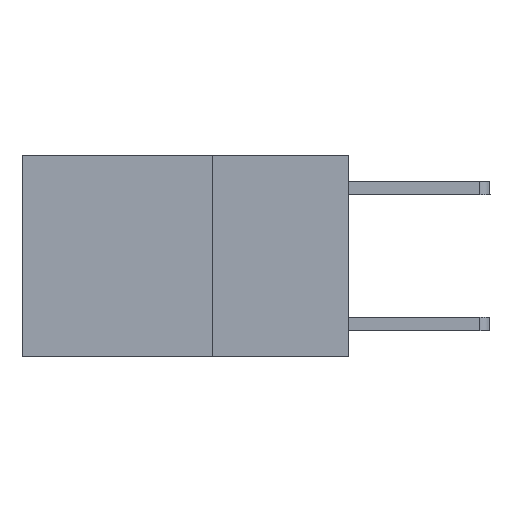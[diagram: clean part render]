
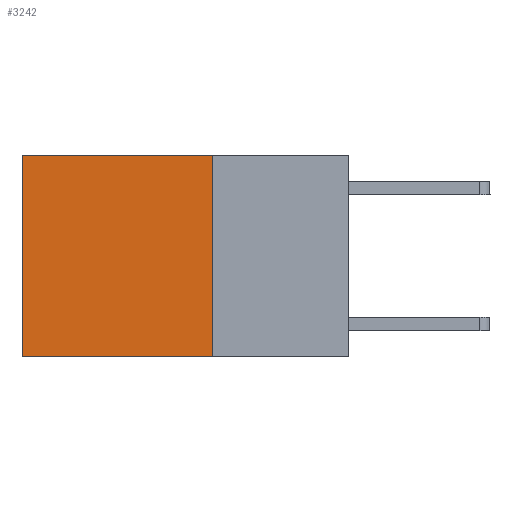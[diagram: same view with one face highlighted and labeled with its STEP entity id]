
A CAD part, left-side view. The second image highlights one B-rep face of the part: STEP entity #3242.
In plain terms, the highlighted planar face has unit normal (-1, 0, 0).
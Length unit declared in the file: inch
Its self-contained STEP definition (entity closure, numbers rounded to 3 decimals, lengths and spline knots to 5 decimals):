
#153 = VECTOR ( 'NONE', #1474, 39.37008 ) ;
#542 = CARTESIAN_POINT ( 'NONE',  ( 0.2625, 0.6, 0. ) ) ;
#686 = VERTEX_POINT ( 'NONE', #6622 ) ;
#793 = EDGE_CURVE ( 'NONE', #686, #1747, #1711, .T. ) ;
#1313 = AXIS2_PLACEMENT_3D ( 'NONE', #2365, #9253, #4961 ) ;
#1388 = LINE ( 'NONE', #542, #5122 ) ;
#1440 = EDGE_CURVE ( 'NONE', #686, #9752, #7326, .T. ) ;
#1474 = DIRECTION ( 'NONE',  ( 0., 1., 0. ) ) ;
#1711 = LINE ( 'NONE', #1775, #5719 ) ;
#1747 = VERTEX_POINT ( 'NONE', #4482 ) ;
#1775 = CARTESIAN_POINT ( 'NONE',  ( 0.2625, 0.25, 0. ) ) ;
#2359 = EDGE_CURVE ( 'NONE', #9752, #10469, #1388, .T. ) ;
#2365 = CARTESIAN_POINT ( 'NONE',  ( 0.2625, 0.25, 0. ) ) ;
#2575 = ORIENTED_EDGE ( 'NONE', *, *, #9671, .F. ) ;
#2678 = ORIENTED_EDGE ( 'NONE', *, *, #793, .F. ) ;
#2779 = DIRECTION ( 'NONE',  ( 0., 0., -1. ) ) ;
#3090 = DIRECTION ( 'NONE',  ( 0., 1., 0. ) ) ;
#3240 = LINE ( 'NONE', #7559, #153 ) ;
#3242 = ADVANCED_FACE ( 'NONE', ( #11192 ), #10095, .F. ) ;
#4482 = CARTESIAN_POINT ( 'NONE',  ( 0.2625, 0.25, -0.37 ) ) ;
#4822 = CARTESIAN_POINT ( 'NONE',  ( 0.2625, 0.25, 0. ) ) ;
#4961 = DIRECTION ( 'NONE',  ( 0., 0., -1. ) ) ;
#5122 = VECTOR ( 'NONE', #2779, 39.37008 ) ;
#5719 = VECTOR ( 'NONE', #6914, 39.37008 ) ;
#6073 = ORIENTED_EDGE ( 'NONE', *, *, #2359, .T. ) ;
#6189 = CARTESIAN_POINT ( 'NONE',  ( 0.2625, 0.6, 0. ) ) ;
#6622 = CARTESIAN_POINT ( 'NONE',  ( 0.2625, 0.25, 0. ) ) ;
#6914 = DIRECTION ( 'NONE',  ( 0., 0., -1. ) ) ;
#7326 = LINE ( 'NONE', #4822, #10365 ) ;
#7559 = CARTESIAN_POINT ( 'NONE',  ( 0.2625, 0.25, -0.37 ) ) ;
#7883 = ORIENTED_EDGE ( 'NONE', *, *, #1440, .T. ) ;
#9253 = DIRECTION ( 'NONE',  ( 1., 0., 0. ) ) ;
#9671 = EDGE_CURVE ( 'NONE', #1747, #10469, #3240, .T. ) ;
#9752 = VERTEX_POINT ( 'NONE', #6189 ) ;
#10095 = PLANE ( 'NONE',  #1313 ) ;
#10365 = VECTOR ( 'NONE', #3090, 39.37008 ) ;
#10469 = VERTEX_POINT ( 'NONE', #11016 ) ;
#10982 = EDGE_LOOP ( 'NONE', ( #6073, #2575, #2678, #7883 ) ) ;
#11016 = CARTESIAN_POINT ( 'NONE',  ( 0.2625, 0.6, -0.37 ) ) ;
#11192 = FACE_OUTER_BOUND ( 'NONE', #10982, .T. ) ;
